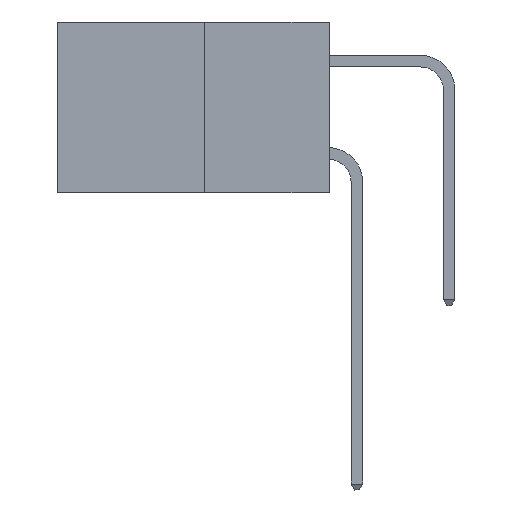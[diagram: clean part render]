
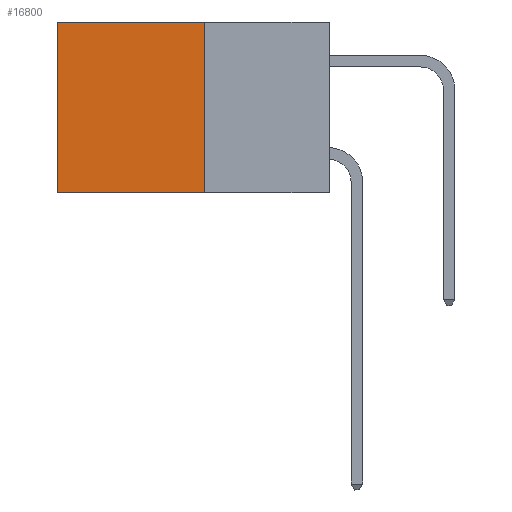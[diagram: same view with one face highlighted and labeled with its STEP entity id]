
A CAD part, left-side view. The second image highlights one B-rep face of the part: STEP entity #16800.
In plain terms, the highlighted planar face has unit normal (-1, 0, 0).
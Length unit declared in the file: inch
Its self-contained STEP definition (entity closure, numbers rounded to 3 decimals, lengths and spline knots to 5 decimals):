
#327 = VECTOR ( 'NONE', #9645, 39.37008 ) ;
#509 = ORIENTED_EDGE ( 'NONE', *, *, #11340, .T. ) ;
#1028 = CARTESIAN_POINT ( 'NONE',  ( 0.277, 0.59, 0. ) ) ;
#2110 = ORIENTED_EDGE ( 'NONE', *, *, #9338, .F. ) ;
#2467 = CARTESIAN_POINT ( 'NONE',  ( 0.277, 0.27, 0. ) ) ;
#2727 = EDGE_CURVE ( 'NONE', #4020, #12598, #11676, .T. ) ;
#3315 = VECTOR ( 'NONE', #25234, 39.37008 ) ;
#4020 = VERTEX_POINT ( 'NONE', #1028 ) ;
#5141 = EDGE_CURVE ( 'NONE', #15860, #12598, #24420, .T. ) ;
#7364 = VECTOR ( 'NONE', #16419, 39.37008 ) ;
#8919 = FACE_OUTER_BOUND ( 'NONE', #15753, .T. ) ;
#9101 = DIRECTION ( 'NONE',  ( 1., 0., 0. ) ) ;
#9338 = EDGE_CURVE ( 'NONE', #15784, #15860, #15577, .T. ) ;
#9645 = DIRECTION ( 'NONE',  ( 0., 0., -1. ) ) ;
#10326 = VECTOR ( 'NONE', #17911, 39.37008 ) ;
#10452 = CARTESIAN_POINT ( 'NONE',  ( 0.277, 0.59, -0.37 ) ) ;
#11340 = EDGE_CURVE ( 'NONE', #15784, #4020, #22558, .T. ) ;
#11676 = LINE ( 'NONE', #10452, #327 ) ;
#12598 = VERTEX_POINT ( 'NONE', #17550 ) ;
#14897 = ORIENTED_EDGE ( 'NONE', *, *, #2727, .T. ) ;
#15530 = ORIENTED_EDGE ( 'NONE', *, *, #5141, .F. ) ;
#15577 = LINE ( 'NONE', #19756, #10326 ) ;
#15753 = EDGE_LOOP ( 'NONE', ( #14897, #15530, #2110, #509 ) ) ;
#15784 = VERTEX_POINT ( 'NONE', #17539 ) ;
#15860 = VERTEX_POINT ( 'NONE', #21724 ) ;
#16419 = DIRECTION ( 'NONE',  ( 0., 1., 0. ) ) ;
#16478 = CARTESIAN_POINT ( 'NONE',  ( 0.277, 0.27, -0.37 ) ) ;
#16800 = ADVANCED_FACE ( 'NONE', ( #8919 ), #20992, .F. ) ;
#17539 = CARTESIAN_POINT ( 'NONE',  ( 0.277, 0.27, 0. ) ) ;
#17550 = CARTESIAN_POINT ( 'NONE',  ( 0.277, 0.59, -0.37 ) ) ;
#17911 = DIRECTION ( 'NONE',  ( 0., 0., -1. ) ) ;
#18714 = AXIS2_PLACEMENT_3D ( 'NONE', #19010, #9101, #22955 ) ;
#19010 = CARTESIAN_POINT ( 'NONE',  ( 0.277, 0.27, -0.37 ) ) ;
#19756 = CARTESIAN_POINT ( 'NONE',  ( 0.277, 0.27, -0.37 ) ) ;
#20992 = PLANE ( 'NONE',  #18714 ) ;
#21724 = CARTESIAN_POINT ( 'NONE',  ( 0.277, 0.27, -0.37 ) ) ;
#22558 = LINE ( 'NONE', #2467, #7364 ) ;
#22955 = DIRECTION ( 'NONE',  ( 0., 0., -1. ) ) ;
#24420 = LINE ( 'NONE', #16478, #3315 ) ;
#25234 = DIRECTION ( 'NONE',  ( 0., 1., 0. ) ) ;
